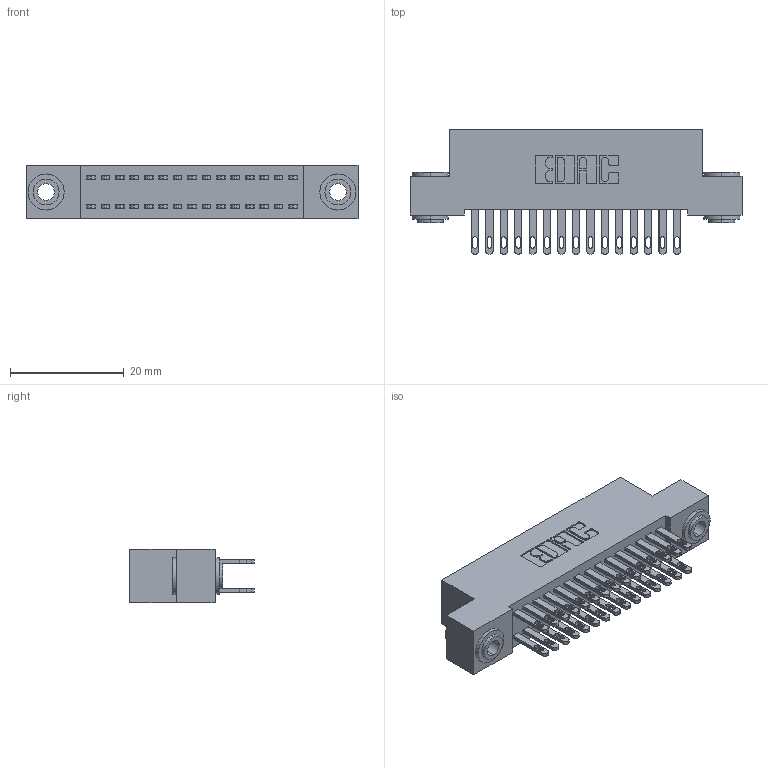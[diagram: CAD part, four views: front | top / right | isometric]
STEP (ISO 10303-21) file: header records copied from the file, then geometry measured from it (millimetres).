
FILE_DESCRIPTION (( 'STEP AP203' ), '1' );
FILE_NAME ('342-030-500-203.STEP', '2019-10-02T04:08:08', ( '' ), ( '' ), 'SwSTEP 2.0', 'SolidWorks 2016', '' );
FILE_SCHEMA (( 'CONFIG_CONTROL_DESIGN' ));
Length unit declared in the file: inch
Products named in the file (4): 342 Part_.156 TH; 345-292-001_345-293-100; 342-250-002_345-250-002-102; 342-030-500-203
Assembly tree (33 placements, depth 2):
  342-030-500-203
    342 Part_.156 TH
    345-292-001_345-293-100  x30
    342-250-002_345-250-002-102  x2
Bounding box: 58.42 x 21.85 x 9.4 mm (x, y, z)
Volume: 5235.7 mm3; surface area: 8358.5 mm2
Topology: 33 solids, 33 shells, 1588 faces, 4785 edges, 3186 vertices
Faces by surface type: plane 976, cylinder 604, cone 8
Entity records: 13590 total; most frequent: CARTESIAN_POINT 2257, ORIENTED_EDGE 2186, DIRECTION 2011, EDGE_CURVE 1093, LINE 937, VECTOR 937, VERTEX_POINT 726, AXIS2_PLACEMENT_3D 537
